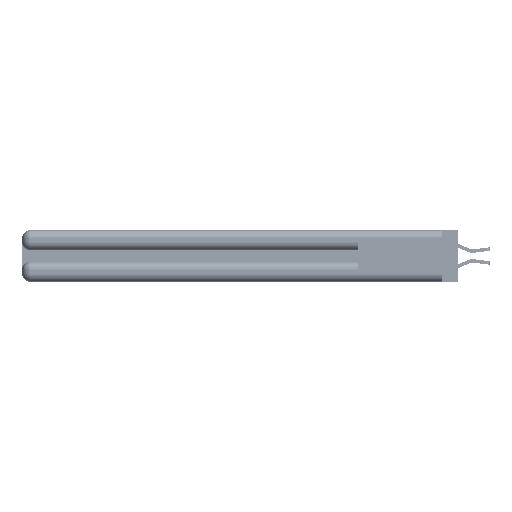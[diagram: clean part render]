
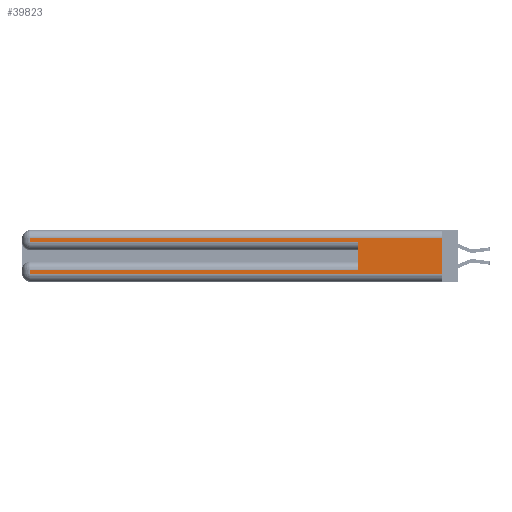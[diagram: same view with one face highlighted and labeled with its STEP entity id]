
A CAD part, left-side view. The second image highlights one B-rep face of the part: STEP entity #39823.
In plain terms, the highlighted planar face has unit normal (-1, 0, 0).
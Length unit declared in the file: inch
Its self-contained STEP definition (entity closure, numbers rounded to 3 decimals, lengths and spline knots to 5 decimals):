
#433 = EDGE_CURVE ( 'NONE', #1828, #20579, #18467, .T. ) ;
#722 = LINE ( 'NONE', #2009, #6427 ) ;
#1287 = CARTESIAN_POINT ( 'NONE',  ( 0., 0.6, 0.285 ) ) ;
#1398 = ORIENTED_EDGE ( 'NONE', *, *, #25547, .T. ) ;
#1417 = CARTESIAN_POINT ( 'NONE',  ( 0., 2.94, 0.31 ) ) ;
#1828 = VERTEX_POINT ( 'NONE', #28272 ) ;
#2009 = CARTESIAN_POINT ( 'NONE',  ( 0., 0., 0.37 ) ) ;
#2669 = VECTOR ( 'NONE', #8082, 39.37008 ) ;
#2670 = ORIENTED_EDGE ( 'NONE', *, *, #35623, .T. ) ;
#5167 = AXIS2_PLACEMENT_3D ( 'NONE', #30128, #38314, #13854 ) ;
#5204 = ORIENTED_EDGE ( 'NONE', *, *, #43537, .T. ) ;
#5358 = CARTESIAN_POINT ( 'NONE',  ( 0., 0.6, 0.145 ) ) ;
#5969 = EDGE_CURVE ( 'NONE', #15745, #20579, #722, .T. ) ;
#6427 = VECTOR ( 'NONE', #10225, 39.37008 ) ;
#6536 = DIRECTION ( 'NONE',  ( 0., 1., 0. ) ) ;
#7081 = CARTESIAN_POINT ( 'NONE',  ( 0., 0., 0.06 ) ) ;
#7870 = EDGE_CURVE ( 'NONE', #47600, #17848, #37011, .T. ) ;
#8035 = CARTESIAN_POINT ( 'NONE',  ( 0., 0., 0.06 ) ) ;
#8082 = DIRECTION ( 'NONE',  ( 0., 0., -1. ) ) ;
#8541 = DIRECTION ( 'NONE',  ( 0., 1., 0. ) ) ;
#8857 = VECTOR ( 'NONE', #35646, 39.37008 ) ;
#9144 = CARTESIAN_POINT ( 'NONE',  ( 0., 2.94, 0.37 ) ) ;
#9761 = PLANE ( 'NONE',  #5167 ) ;
#9825 = DIRECTION ( 'NONE',  ( 0., -1., 0. ) ) ;
#10225 = DIRECTION ( 'NONE',  ( 0., 0., -1. ) ) ;
#10364 = ORIENTED_EDGE ( 'NONE', *, *, #433, .T. ) ;
#11381 = LINE ( 'NONE', #9144, #41404 ) ;
#12223 = CARTESIAN_POINT ( 'NONE',  ( 0., 2.94, 0.285 ) ) ;
#12530 = EDGE_LOOP ( 'NONE', ( #42268, #1398, #2670, #5204, #26997, #51258, #30816, #10364 ) ) ;
#13446 = DIRECTION ( 'NONE',  ( 0., 0., -1. ) ) ;
#13854 = DIRECTION ( 'NONE',  ( 0., 0., -1. ) ) ;
#14482 = CARTESIAN_POINT ( 'NONE',  ( 0., 2.94, 0.085 ) ) ;
#15255 = VECTOR ( 'NONE', #33943, 39.37008 ) ;
#15745 = VERTEX_POINT ( 'NONE', #23254 ) ;
#17848 = VERTEX_POINT ( 'NONE', #1287 ) ;
#18256 = EDGE_CURVE ( 'NONE', #47600, #48622, #25114, .T. ) ;
#18414 = VERTEX_POINT ( 'NONE', #1417 ) ;
#18467 = LINE ( 'NONE', #7081, #8857 ) ;
#20579 = VERTEX_POINT ( 'NONE', #8035 ) ;
#23254 = CARTESIAN_POINT ( 'NONE',  ( 0., 0., 0.31 ) ) ;
#23621 = VECTOR ( 'NONE', #6536, 39.37008 ) ;
#25114 = LINE ( 'NONE', #41229, #33357 ) ;
#25547 = EDGE_CURVE ( 'NONE', #15745, #18414, #46601, .T. ) ;
#26951 = CARTESIAN_POINT ( 'NONE',  ( 0., 0., 0.31 ) ) ;
#26997 = ORIENTED_EDGE ( 'NONE', *, *, #7870, .F. ) ;
#28272 = CARTESIAN_POINT ( 'NONE',  ( 0., 2.94, 0.06 ) ) ;
#28483 = CARTESIAN_POINT ( 'NONE',  ( 0., 2.94, 0.37 ) ) ;
#30128 = CARTESIAN_POINT ( 'NONE',  ( 0., 0., 0.37 ) ) ;
#30816 = ORIENTED_EDGE ( 'NONE', *, *, #46470, .T. ) ;
#33357 = VECTOR ( 'NONE', #8541, 39.37008 ) ;
#33943 = DIRECTION ( 'NONE',  ( 0., 0., 1. ) ) ;
#33948 = VECTOR ( 'NONE', #9825, 39.37008 ) ;
#35623 = EDGE_CURVE ( 'NONE', #18414, #35630, #36534, .T. ) ;
#35630 = VERTEX_POINT ( 'NONE', #12223 ) ;
#35646 = DIRECTION ( 'NONE',  ( 0., -1., 0. ) ) ;
#36534 = LINE ( 'NONE', #28483, #2669 ) ;
#37011 = LINE ( 'NONE', #5358, #15255 ) ;
#38314 = DIRECTION ( 'NONE',  ( 1., 0., 0. ) ) ;
#39823 = ADVANCED_FACE ( 'NONE', ( #46643 ), #9761, .F. ) ;
#40633 = CARTESIAN_POINT ( 'NONE',  ( 0., 0.6, 0.085 ) ) ;
#41229 = CARTESIAN_POINT ( 'NONE',  ( 0., 0., 0.085 ) ) ;
#41404 = VECTOR ( 'NONE', #13446, 39.37008 ) ;
#42268 = ORIENTED_EDGE ( 'NONE', *, *, #5969, .F. ) ;
#43537 = EDGE_CURVE ( 'NONE', #35630, #17848, #44830, .T. ) ;
#44830 = LINE ( 'NONE', #50566, #33948 ) ;
#46470 = EDGE_CURVE ( 'NONE', #48622, #1828, #11381, .T. ) ;
#46601 = LINE ( 'NONE', #26951, #23621 ) ;
#46643 = FACE_OUTER_BOUND ( 'NONE', #12530, .T. ) ;
#47600 = VERTEX_POINT ( 'NONE', #40633 ) ;
#48622 = VERTEX_POINT ( 'NONE', #14482 ) ;
#50566 = CARTESIAN_POINT ( 'NONE',  ( 0., 0., 0.285 ) ) ;
#51258 = ORIENTED_EDGE ( 'NONE', *, *, #18256, .T. ) ;
